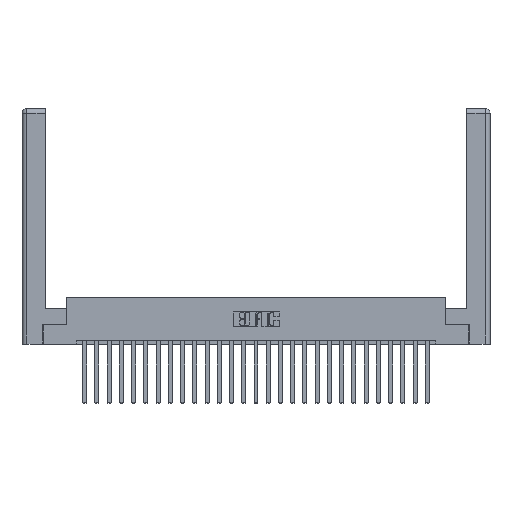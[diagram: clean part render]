
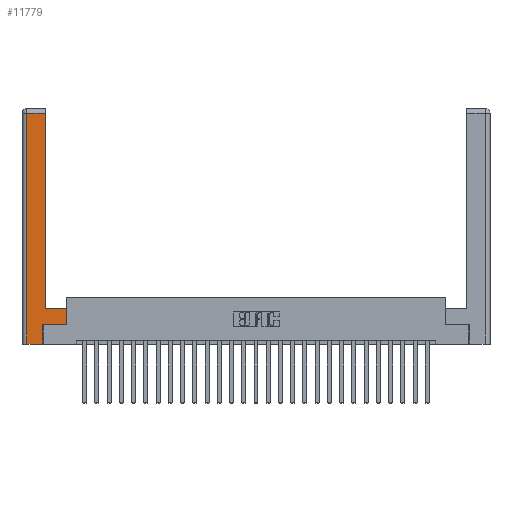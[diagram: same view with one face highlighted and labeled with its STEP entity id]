
A CAD part, top view. The second image highlights one B-rep face of the part: STEP entity #11779.
In plain terms, the highlighted planar face has unit normal (0, 0, 1).
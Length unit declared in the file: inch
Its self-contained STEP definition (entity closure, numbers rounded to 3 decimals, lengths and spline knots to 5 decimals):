
#296 = FACE_OUTER_BOUND ( 'NONE', #14293, .T. ) ;
#740 = VERTEX_POINT ( 'NONE', #6458 ) ;
#772 = AXIS2_PLACEMENT_3D ( 'NONE', #15573, #9291, #9480 ) ;
#821 = CARTESIAN_POINT ( 'NONE',  ( 0.0615, 0., 0. ) ) ;
#1460 = ORIENTED_EDGE ( 'NONE', *, *, #12188, .T. ) ;
#1522 = VECTOR ( 'NONE', #5403, 39.37008 ) ;
#1562 = ORIENTED_EDGE ( 'NONE', *, *, #18676, .T. ) ;
#1570 = DIRECTION ( 'NONE',  ( 0., 1., 0. ) ) ;
#1621 = CARTESIAN_POINT ( 'NONE',  ( 0.565, 0.245, 0. ) ) ;
#2125 = CARTESIAN_POINT ( 'NONE',  ( 0.295, 2.94, 0. ) ) ;
#2336 = VERTEX_POINT ( 'NONE', #8843 ) ;
#2876 = VECTOR ( 'NONE', #1570, 39.37008 ) ;
#4220 = DIRECTION ( 'NONE',  ( 1., 0., 0. ) ) ;
#4340 = CARTESIAN_POINT ( 'NONE',  ( 0.265, 0.245, 0. ) ) ;
#4718 = LINE ( 'NONE', #14534, #25934 ) ;
#4980 = DIRECTION ( 'NONE',  ( 0., -1., 0. ) ) ;
#5403 = DIRECTION ( 'NONE',  ( 1., 0., 0. ) ) ;
#5544 = CARTESIAN_POINT ( 'NONE',  ( 0.0615, 2.94, 0. ) ) ;
#6175 = VERTEX_POINT ( 'NONE', #11023 ) ;
#6458 = CARTESIAN_POINT ( 'NONE',  ( 0.565, 0.45, 0. ) ) ;
#6777 = LINE ( 'NONE', #11891, #13591 ) ;
#7623 = DIRECTION ( 'NONE',  ( -1., 0., 0. ) ) ;
#7901 = VECTOR ( 'NONE', #4980, 39.37008 ) ;
#8769 = VERTEX_POINT ( 'NONE', #2125 ) ;
#8843 = CARTESIAN_POINT ( 'NONE',  ( 0.295, 0.45, 0. ) ) ;
#8845 = ORIENTED_EDGE ( 'NONE', *, *, #14882, .T. ) ;
#8899 = CARTESIAN_POINT ( 'NONE',  ( 0.565, 0.245, 0. ) ) ;
#9223 = LINE ( 'NONE', #22141, #16080 ) ;
#9291 = DIRECTION ( 'NONE',  ( 0., 0., -1. ) ) ;
#9480 = DIRECTION ( 'NONE',  ( -1., 0., 0. ) ) ;
#9508 = VERTEX_POINT ( 'NONE', #8899 ) ;
#9657 = VECTOR ( 'NONE', #20883, 39.37008 ) ;
#10940 = VERTEX_POINT ( 'NONE', #16063 ) ;
#11023 = CARTESIAN_POINT ( 'NONE',  ( 0.265, 0.245, 0. ) ) ;
#11420 = EDGE_CURVE ( 'NONE', #740, #2336, #6777, .T. ) ;
#11779 = ADVANCED_FACE ( 'NONE', ( #296 ), #21612, .F. ) ;
#11891 = CARTESIAN_POINT ( 'NONE',  ( 0.295, 0.45, 0. ) ) ;
#12188 = EDGE_CURVE ( 'NONE', #10940, #6175, #13214, .T. ) ;
#12193 = DIRECTION ( 'NONE',  ( 0., 1., 0. ) ) ;
#13214 = LINE ( 'NONE', #4340, #9657 ) ;
#13424 = EDGE_CURVE ( 'NONE', #2336, #8769, #18696, .T. ) ;
#13591 = VECTOR ( 'NONE', #7623, 39.37008 ) ;
#13803 = LINE ( 'NONE', #1621, #1522 ) ;
#13945 = CARTESIAN_POINT ( 'NONE',  ( 0.295, 3., 0. ) ) ;
#14293 = EDGE_LOOP ( 'NONE', ( #22073, #20602, #17550, #22107, #1460, #1562, #8845, #26364 ) ) ;
#14534 = CARTESIAN_POINT ( 'NONE',  ( 0.265, 0., 0. ) ) ;
#14882 = EDGE_CURVE ( 'NONE', #9508, #740, #9223, .T. ) ;
#15573 = CARTESIAN_POINT ( 'NONE',  ( 0., 0., 0. ) ) ;
#15574 = VERTEX_POINT ( 'NONE', #23279 ) ;
#15828 = CARTESIAN_POINT ( 'NONE',  ( 0.0615, 2.94, 0. ) ) ;
#15867 = EDGE_CURVE ( 'NONE', #8769, #19942, #21730, .T. ) ;
#16063 = CARTESIAN_POINT ( 'NONE',  ( 0.265, 0., 0. ) ) ;
#16080 = VECTOR ( 'NONE', #12193, 39.37008 ) ;
#17550 = ORIENTED_EDGE ( 'NONE', *, *, #24992, .T. ) ;
#17918 = LINE ( 'NONE', #821, #7901 ) ;
#18250 = VECTOR ( 'NONE', #26089, 39.37008 ) ;
#18676 = EDGE_CURVE ( 'NONE', #6175, #9508, #13803, .T. ) ;
#18696 = LINE ( 'NONE', #13945, #2876 ) ;
#19094 = EDGE_CURVE ( 'NONE', #15574, #10940, #4718, .T. ) ;
#19942 = VERTEX_POINT ( 'NONE', #5544 ) ;
#20602 = ORIENTED_EDGE ( 'NONE', *, *, #15867, .T. ) ;
#20883 = DIRECTION ( 'NONE',  ( 0., 1., 0. ) ) ;
#21612 = PLANE ( 'NONE',  #772 ) ;
#21730 = LINE ( 'NONE', #15828, #18250 ) ;
#22073 = ORIENTED_EDGE ( 'NONE', *, *, #13424, .T. ) ;
#22107 = ORIENTED_EDGE ( 'NONE', *, *, #19094, .T. ) ;
#22141 = CARTESIAN_POINT ( 'NONE',  ( 0.565, 0.45, 0. ) ) ;
#23279 = CARTESIAN_POINT ( 'NONE',  ( 0.0615, 0., 0. ) ) ;
#24992 = EDGE_CURVE ( 'NONE', #19942, #15574, #17918, .T. ) ;
#25934 = VECTOR ( 'NONE', #4220, 39.37008 ) ;
#26089 = DIRECTION ( 'NONE',  ( -1., 0., 0. ) ) ;
#26364 = ORIENTED_EDGE ( 'NONE', *, *, #11420, .T. ) ;
